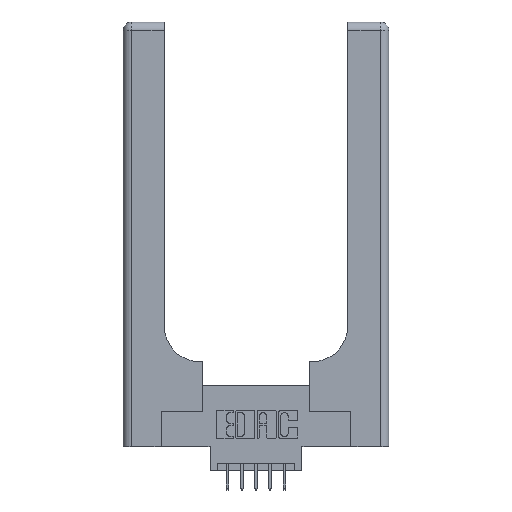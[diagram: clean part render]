
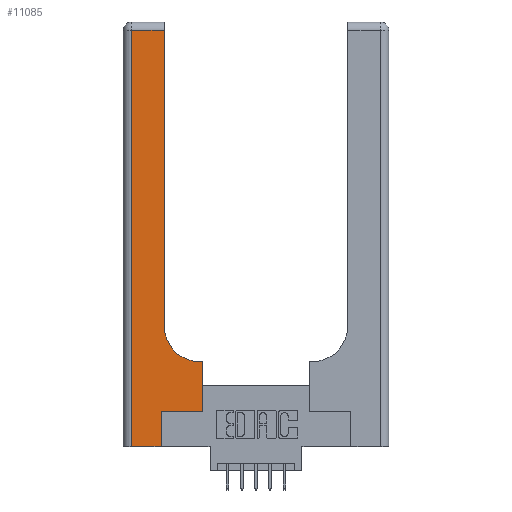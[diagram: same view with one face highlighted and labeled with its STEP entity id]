
A CAD part, top view. The second image highlights one B-rep face of the part: STEP entity #11085.
In plain terms, the highlighted planar face has unit normal (0, 0, 1).
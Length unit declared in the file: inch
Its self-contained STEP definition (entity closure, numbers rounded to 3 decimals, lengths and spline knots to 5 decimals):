
#32 = VERTEX_POINT ( 'NONE', #2724 ) ;
#123 = VECTOR ( 'NONE', #1467, 39.37008 ) ;
#208 = EDGE_CURVE ( 'NONE', #32, #3161, #8363, .T. ) ;
#210 = VERTEX_POINT ( 'NONE', #9808 ) ;
#310 = LINE ( 'NONE', #5871, #9339 ) ;
#347 = CARTESIAN_POINT ( 'NONE',  ( 0.5415, 0.85, 0.37 ) ) ;
#579 = VERTEX_POINT ( 'NONE', #10671 ) ;
#676 = CARTESIAN_POINT ( 'NONE',  ( 0.5585, 0.6, 0.37 ) ) ;
#781 = DIRECTION ( 'NONE',  ( 0., 1., 0. ) ) ;
#803 = ORIENTED_EDGE ( 'NONE', *, *, #6434, .T. ) ;
#940 = VECTOR ( 'NONE', #9544, 39.37008 ) ;
#1001 = EDGE_CURVE ( 'NONE', #579, #4320, #7493, .T. ) ;
#1226 = DIRECTION ( 'NONE',  ( 0., 0., -1. ) ) ;
#1326 = VERTEX_POINT ( 'NONE', #6776 ) ;
#1398 = LINE ( 'NONE', #4923, #10000 ) ;
#1467 = DIRECTION ( 'NONE',  ( 0., 1., 0. ) ) ;
#1782 = ORIENTED_EDGE ( 'NONE', *, *, #13349, .T. ) ;
#1936 = EDGE_CURVE ( 'NONE', #4571, #8813, #12966, .T. ) ;
#2108 = VECTOR ( 'NONE', #781, 39.37008 ) ;
#2195 = CARTESIAN_POINT ( 'NONE',  ( 0.06, 3., 0.37 ) ) ;
#2227 = CARTESIAN_POINT ( 'NONE',  ( 0.2915, 2.94, 0.37 ) ) ;
#2316 = CARTESIAN_POINT ( 'NONE',  ( 0., 3., 0.37 ) ) ;
#2360 = CARTESIAN_POINT ( 'NONE',  ( 0.06, 0., 0.37 ) ) ;
#2529 = DIRECTION ( 'NONE',  ( 1., 0., 0. ) ) ;
#2724 = CARTESIAN_POINT ( 'NONE',  ( 0.06, 2.94, 0.37 ) ) ;
#2961 = CARTESIAN_POINT ( 'NONE',  ( 0., 0., 0.37 ) ) ;
#3079 = CARTESIAN_POINT ( 'NONE',  ( 0.269, 0., 0.37 ) ) ;
#3112 = ORIENTED_EDGE ( 'NONE', *, *, #8980, .T. ) ;
#3161 = VERTEX_POINT ( 'NONE', #2360 ) ;
#3476 = VECTOR ( 'NONE', #5204, 39.37008 ) ;
#4320 = VERTEX_POINT ( 'NONE', #5303 ) ;
#4514 = CARTESIAN_POINT ( 'NONE',  ( 0.5415, 0.6, 0.37 ) ) ;
#4534 = PLANE ( 'NONE',  #12617 ) ;
#4571 = VERTEX_POINT ( 'NONE', #676 ) ;
#4700 = DIRECTION ( 'NONE',  ( 1., 0., 0. ) ) ;
#4782 = DIRECTION ( 'NONE',  ( -1., 0., 0. ) ) ;
#4923 = CARTESIAN_POINT ( 'NONE',  ( 0., 2.94, 0.37 ) ) ;
#5204 = DIRECTION ( 'NONE',  ( -1., 0., 0. ) ) ;
#5303 = CARTESIAN_POINT ( 'NONE',  ( 0.269, 0.25, 0.37 ) ) ;
#5730 = ORIENTED_EDGE ( 'NONE', *, *, #7202, .T. ) ;
#5871 = CARTESIAN_POINT ( 'NONE',  ( 0.269, 0.25, 0.37 ) ) ;
#5954 = VERTEX_POINT ( 'NONE', #2227 ) ;
#6174 = ORIENTED_EDGE ( 'NONE', *, *, #1001, .T. ) ;
#6310 = ORIENTED_EDGE ( 'NONE', *, *, #1936, .T. ) ;
#6434 = EDGE_CURVE ( 'NONE', #1326, #4571, #12348, .T. ) ;
#6716 = DIRECTION ( 'NONE',  ( -1., 0., 0. ) ) ;
#6776 = CARTESIAN_POINT ( 'NONE',  ( 0.5585, 0.25, 0.37 ) ) ;
#7202 = EDGE_CURVE ( 'NONE', #8813, #210, #11703, .T. ) ;
#7493 = LINE ( 'NONE', #3079, #2108 ) ;
#7599 = ORIENTED_EDGE ( 'NONE', *, *, #7606, .T. ) ;
#7606 = EDGE_CURVE ( 'NONE', #5954, #32, #1398, .T. ) ;
#7809 = FACE_OUTER_BOUND ( 'NONE', #11119, .T. ) ;
#8031 = ORIENTED_EDGE ( 'NONE', *, *, #12016, .T. ) ;
#8054 = CARTESIAN_POINT ( 'NONE',  ( 0.5585, 0.25, 0.37 ) ) ;
#8363 = LINE ( 'NONE', #2195, #940 ) ;
#8404 = DIRECTION ( 'NONE',  ( 1., 0., 0. ) ) ;
#8813 = VERTEX_POINT ( 'NONE', #4514 ) ;
#8980 = EDGE_CURVE ( 'NONE', #4320, #1326, #310, .T. ) ;
#9339 = VECTOR ( 'NONE', #4700, 39.37008 ) ;
#9544 = DIRECTION ( 'NONE',  ( 0., -1., 0. ) ) ;
#9808 = CARTESIAN_POINT ( 'NONE',  ( 0.2915, 0.85, 0.37 ) ) ;
#10000 = VECTOR ( 'NONE', #4782, 39.37008 ) ;
#10534 = LINE ( 'NONE', #2961, #11021 ) ;
#10671 = CARTESIAN_POINT ( 'NONE',  ( 0.269, 0., 0.37 ) ) ;
#11021 = VECTOR ( 'NONE', #8404, 39.37008 ) ;
#11085 = ADVANCED_FACE ( 'NONE', ( #7809 ), #4534, .F. ) ;
#11119 = EDGE_LOOP ( 'NONE', ( #1782, #7599, #12010, #8031, #6174, #3112, #803, #6310, #5730 ) ) ;
#11703 = CIRCLE ( 'NONE', #12848, 0.25 ) ;
#12010 = ORIENTED_EDGE ( 'NONE', *, *, #208, .T. ) ;
#12016 = EDGE_CURVE ( 'NONE', #3161, #579, #10534, .T. ) ;
#12167 = CARTESIAN_POINT ( 'NONE',  ( 0.2915, 3., 0.37 ) ) ;
#12348 = LINE ( 'NONE', #8054, #123 ) ;
#12617 = AXIS2_PLACEMENT_3D ( 'NONE', #2316, #1226, #6716 ) ;
#12848 = AXIS2_PLACEMENT_3D ( 'NONE', #347, #13662, #2529 ) ;
#12909 = CARTESIAN_POINT ( 'NONE',  ( 0.2915, 0.6, 0.37 ) ) ;
#12966 = LINE ( 'NONE', #12909, #3476 ) ;
#13098 = LINE ( 'NONE', #12167, #13114 ) ;
#13114 = VECTOR ( 'NONE', #13310, 39.37008 ) ;
#13310 = DIRECTION ( 'NONE',  ( 0., 1., 0. ) ) ;
#13349 = EDGE_CURVE ( 'NONE', #210, #5954, #13098, .T. ) ;
#13662 = DIRECTION ( 'NONE',  ( 0., 0., -1. ) ) ;
